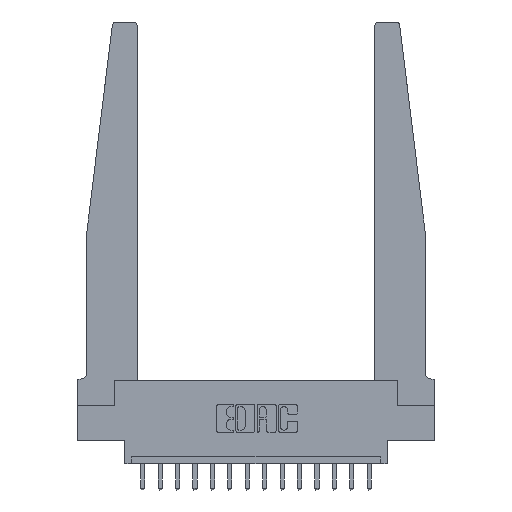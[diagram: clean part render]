
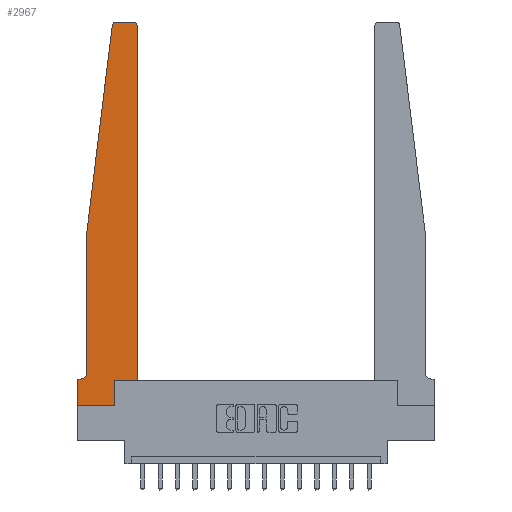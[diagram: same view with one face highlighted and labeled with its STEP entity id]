
A CAD part, top view. The second image highlights one B-rep face of the part: STEP entity #2967.
In plain terms, the highlighted planar face has unit normal (0, 0, 1).
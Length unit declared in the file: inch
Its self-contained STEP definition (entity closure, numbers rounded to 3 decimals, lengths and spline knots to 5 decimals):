
#5 = VERTEX_POINT ( 'NONE', #2515 ) ;
#27 = ORIENTED_EDGE ( 'NONE', *, *, #8765, .T. ) ;
#74 = EDGE_CURVE ( 'NONE', #5055, #7908, #6632, .T. ) ;
#350 = CARTESIAN_POINT ( 'NONE',  ( 0.25, 2.75, 0.37 ) ) ;
#616 = DIRECTION ( 'NONE',  ( 0., 0., 1. ) ) ;
#619 = EDGE_LOOP ( 'NONE', ( #16903, #27, #7267, #10698, #11547, #13551, #15198, #2184, #8248, #3344, #9433, #3452 ) ) ;
#637 = AXIS2_PLACEMENT_3D ( 'NONE', #5483, #5598, #15059 ) ;
#786 = CARTESIAN_POINT ( 'NONE',  ( 0.395, 2.72, 0.37 ) ) ;
#840 = DIRECTION ( 'NONE',  ( 1., 0., 0. ) ) ;
#892 = VECTOR ( 'NONE', #10962, 39.37008 ) ;
#1219 = DIRECTION ( 'NONE',  ( 0., -1., 0. ) ) ;
#1256 = CARTESIAN_POINT ( 'NONE',  ( 0.065, 0.2375, 0.37 ) ) ;
#1380 = PLANE ( 'NONE',  #637 ) ;
#1501 = VECTOR ( 'NONE', #8614, 39.37008 ) ;
#1534 = VECTOR ( 'NONE', #10352, 39.37008 ) ;
#1662 = AXIS2_PLACEMENT_3D ( 'NONE', #15094, #7548, #4006 ) ;
#1883 = DIRECTION ( 'NONE',  ( 0., -1., 0. ) ) ;
#2129 = EDGE_CURVE ( 'NONE', #7908, #7969, #7426, .T. ) ;
#2184 = ORIENTED_EDGE ( 'NONE', *, *, #9156, .T. ) ;
#2211 = VERTEX_POINT ( 'NONE', #3147 ) ;
#2231 = LINE ( 'NONE', #15007, #12535 ) ;
#2449 = CARTESIAN_POINT ( 'NONE',  ( 0.065, 1.25, 0.37 ) ) ;
#2515 = CARTESIAN_POINT ( 'NONE',  ( 0.2605, 0., 0.37 ) ) ;
#2946 = CARTESIAN_POINT ( 'NONE',  ( 0.425, 0.18, 0.37 ) ) ;
#2967 = ADVANCED_FACE ( 'NONE', ( #13746 ), #1380, .T. ) ;
#2994 = VECTOR ( 'NONE', #1219, 39.37008 ) ;
#3147 = CARTESIAN_POINT ( 'NONE',  ( 0., 0., 0.37 ) ) ;
#3344 = ORIENTED_EDGE ( 'NONE', *, *, #5218, .T. ) ;
#3452 = ORIENTED_EDGE ( 'NONE', *, *, #15474, .T. ) ;
#3528 = EDGE_CURVE ( 'NONE', #7969, #6167, #9828, .T. ) ;
#3561 = DIRECTION ( 'NONE',  ( 1., 0., 0. ) ) ;
#3662 = CARTESIAN_POINT ( 'NONE',  ( 0.425, 0.18, 0.37 ) ) ;
#4006 = DIRECTION ( 'NONE',  ( -1., 0., 0. ) ) ;
#4012 = LINE ( 'NONE', #2946, #1501 ) ;
#4377 = LINE ( 'NONE', #12691, #10899 ) ;
#4720 = VERTEX_POINT ( 'NONE', #6535 ) ;
#5004 = CIRCLE ( 'NONE', #13006, 0.03 ) ;
#5055 = VERTEX_POINT ( 'NONE', #12865 ) ;
#5218 = EDGE_CURVE ( 'NONE', #10943, #4720, #7866, .T. ) ;
#5415 = LINE ( 'NONE', #6825, #14518 ) ;
#5483 = CARTESIAN_POINT ( 'NONE',  ( 0., 0.1875, 0.37 ) ) ;
#5520 = LINE ( 'NONE', #13007, #1534 ) ;
#5557 = DIRECTION ( 'NONE',  ( -0.122, -0.992, 0. ) ) ;
#5598 = DIRECTION ( 'NONE',  ( 0., 0., 1. ) ) ;
#5787 = VERTEX_POINT ( 'NONE', #17405 ) ;
#6167 = VERTEX_POINT ( 'NONE', #12477 ) ;
#6199 = EDGE_CURVE ( 'NONE', #9527, #8663, #6749, .T. ) ;
#6452 = CARTESIAN_POINT ( 'NONE',  ( 0.2605, 0.18, 0.37 ) ) ;
#6535 = CARTESIAN_POINT ( 'NONE',  ( 0.425, 0.18, 0.37 ) ) ;
#6632 = LINE ( 'NONE', #12218, #12774 ) ;
#6749 = LINE ( 'NONE', #350, #892 ) ;
#6825 = CARTESIAN_POINT ( 'NONE',  ( 0.2605, 0.18, 0.37 ) ) ;
#6998 = EDGE_CURVE ( 'NONE', #4720, #5787, #4012, .T. ) ;
#7267 = ORIENTED_EDGE ( 'NONE', *, *, #74, .T. ) ;
#7426 = LINE ( 'NONE', #7967, #2994 ) ;
#7497 = DIRECTION ( 'NONE',  ( 1., 0., 0. ) ) ;
#7548 = DIRECTION ( 'NONE',  ( 0., 0., -1. ) ) ;
#7866 = LINE ( 'NONE', #3662, #8951 ) ;
#7908 = VERTEX_POINT ( 'NONE', #2449 ) ;
#7967 = CARTESIAN_POINT ( 'NONE',  ( 0.065, 1.25, 0.37 ) ) ;
#7969 = VERTEX_POINT ( 'NONE', #1256 ) ;
#8014 = DIRECTION ( 'NONE',  ( 0., 1., 0. ) ) ;
#8248 = ORIENTED_EDGE ( 'NONE', *, *, #15263, .T. ) ;
#8614 = DIRECTION ( 'NONE',  ( 0., 1., 0. ) ) ;
#8663 = VERTEX_POINT ( 'NONE', #15337 ) ;
#8765 = EDGE_CURVE ( 'NONE', #8663, #5055, #5004, .T. ) ;
#8951 = VECTOR ( 'NONE', #3561, 39.37008 ) ;
#9156 = EDGE_CURVE ( 'NONE', #2211, #5, #4377, .T. ) ;
#9433 = ORIENTED_EDGE ( 'NONE', *, *, #6998, .T. ) ;
#9527 = VERTEX_POINT ( 'NONE', #11016 ) ;
#9828 = CIRCLE ( 'NONE', #1662, 0.05 ) ;
#10141 = CARTESIAN_POINT ( 'NONE',  ( 0., 0.1875, 0.37 ) ) ;
#10352 = DIRECTION ( 'NONE',  ( -1., 0., 0. ) ) ;
#10466 = EDGE_CURVE ( 'NONE', #12882, #2211, #2231, .T. ) ;
#10503 = DIRECTION ( 'NONE',  ( 0., 0., 1. ) ) ;
#10695 = CIRCLE ( 'NONE', #11769, 0.03 ) ;
#10698 = ORIENTED_EDGE ( 'NONE', *, *, #2129, .T. ) ;
#10899 = VECTOR ( 'NONE', #7497, 39.37008 ) ;
#10943 = VERTEX_POINT ( 'NONE', #6452 ) ;
#10962 = DIRECTION ( 'NONE',  ( -1., 0., 0. ) ) ;
#11016 = CARTESIAN_POINT ( 'NONE',  ( 0.395, 2.75, 0.37 ) ) ;
#11409 = EDGE_CURVE ( 'NONE', #6167, #12882, #5520, .T. ) ;
#11547 = ORIENTED_EDGE ( 'NONE', *, *, #3528, .T. ) ;
#11769 = AXIS2_PLACEMENT_3D ( 'NONE', #786, #616, #14303 ) ;
#12218 = CARTESIAN_POINT ( 'NONE',  ( 0.065, 1.25, 0.37 ) ) ;
#12477 = CARTESIAN_POINT ( 'NONE',  ( 0.015, 0.1875, 0.37 ) ) ;
#12535 = VECTOR ( 'NONE', #1883, 39.37008 ) ;
#12691 = CARTESIAN_POINT ( 'NONE',  ( 0., 0., 0.37 ) ) ;
#12774 = VECTOR ( 'NONE', #5557, 39.37008 ) ;
#12865 = CARTESIAN_POINT ( 'NONE',  ( 0.24675, 2.72367, 0.37 ) ) ;
#12882 = VERTEX_POINT ( 'NONE', #10141 ) ;
#13006 = AXIS2_PLACEMENT_3D ( 'NONE', #15794, #10503, #840 ) ;
#13007 = CARTESIAN_POINT ( 'NONE',  ( 0.065, 0.1875, 0.37 ) ) ;
#13551 = ORIENTED_EDGE ( 'NONE', *, *, #11409, .T. ) ;
#13746 = FACE_OUTER_BOUND ( 'NONE', #619, .T. ) ;
#14303 = DIRECTION ( 'NONE',  ( 1., 0., 0. ) ) ;
#14518 = VECTOR ( 'NONE', #8014, 39.37008 ) ;
#15007 = CARTESIAN_POINT ( 'NONE',  ( 0., 0., 0.37 ) ) ;
#15059 = DIRECTION ( 'NONE',  ( 1., 0., 0. ) ) ;
#15094 = CARTESIAN_POINT ( 'NONE',  ( 0.015, 0.2375, 0.37 ) ) ;
#15198 = ORIENTED_EDGE ( 'NONE', *, *, #10466, .T. ) ;
#15263 = EDGE_CURVE ( 'NONE', #5, #10943, #5415, .T. ) ;
#15337 = CARTESIAN_POINT ( 'NONE',  ( 0.27653, 2.75, 0.37 ) ) ;
#15474 = EDGE_CURVE ( 'NONE', #5787, #9527, #10695, .T. ) ;
#15794 = CARTESIAN_POINT ( 'NONE',  ( 0.27653, 2.72, 0.37 ) ) ;
#16903 = ORIENTED_EDGE ( 'NONE', *, *, #6199, .T. ) ;
#17405 = CARTESIAN_POINT ( 'NONE',  ( 0.425, 2.72, 0.37 ) ) ;
